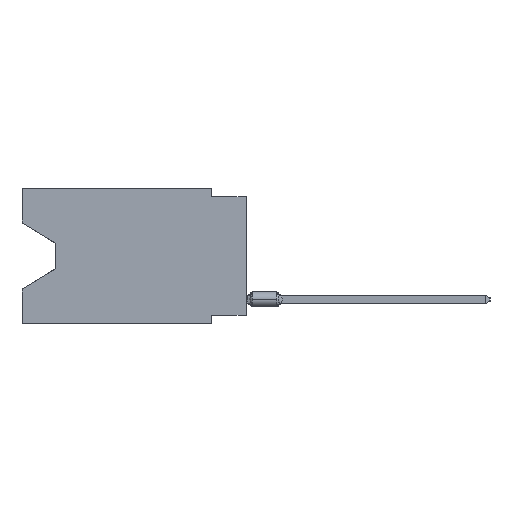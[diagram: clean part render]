
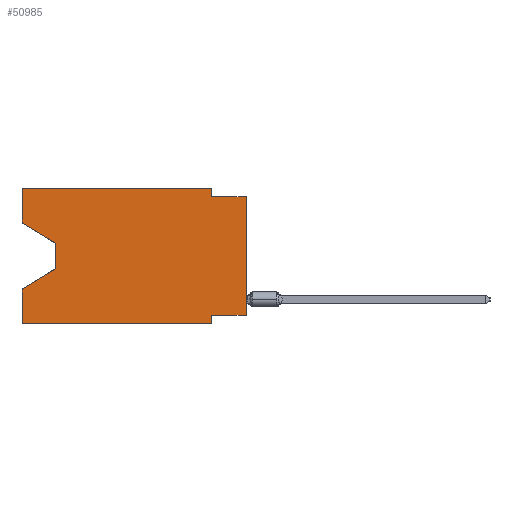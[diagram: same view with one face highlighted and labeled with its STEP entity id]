
A CAD part, left-side view. The second image highlights one B-rep face of the part: STEP entity #50985.
In plain terms, the highlighted planar face has unit normal (-1, 0, 0).
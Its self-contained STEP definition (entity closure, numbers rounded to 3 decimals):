
#1120 = CARTESIAN_POINT ( 'NONE',  ( 0., 0., -9.271 ) ) ;
#1254 = CARTESIAN_POINT ( 'NONE',  ( 0., 13.97, -4.013 ) ) ;
#1329 = EDGE_CURVE ( 'NONE', #47674, #13410, #23877, .T. ) ;
#2119 = EDGE_CURVE ( 'NONE', #50787, #13418, #16677, .T. ) ;
#3861 = EDGE_CURVE ( 'NONE', #7857, #56292, #45244, .T. ) ;
#4808 = VERTEX_POINT ( 'NONE', #8250 ) ;
#4958 = LINE ( 'NONE', #19090, #44811 ) ;
#6176 = ORIENTED_EDGE ( 'NONE', *, *, #52317, .T. ) ;
#6295 = DIRECTION ( 'NONE',  ( 0., 0., -1. ) ) ;
#6825 = VECTOR ( 'NONE', #29955, 1000. ) ;
#6842 = VECTOR ( 'NONE', #49195, 1000. ) ;
#7322 = DIRECTION ( 'NONE',  ( 0., -1., 0. ) ) ;
#7857 = VERTEX_POINT ( 'NONE', #1254 ) ;
#8250 = CARTESIAN_POINT ( 'NONE',  ( 0., 16.383, -7.36 ) ) ;
#8367 = CARTESIAN_POINT ( 'NONE',  ( 0., 16.383, 0. ) ) ;
#8553 = EDGE_CURVE ( 'NONE', #48739, #59104, #13150, .T. ) ;
#12864 = CARTESIAN_POINT ( 'NONE',  ( 0., 2.54, -9.906 ) ) ;
#13150 = LINE ( 'NONE', #26350, #45470 ) ;
#13410 = VERTEX_POINT ( 'NONE', #18545 ) ;
#13416 = EDGE_CURVE ( 'NONE', #17026, #50787, #36682, .T. ) ;
#13418 = VERTEX_POINT ( 'NONE', #55696 ) ;
#13760 = ORIENTED_EDGE ( 'NONE', *, *, #13416, .F. ) ;
#14094 = ORIENTED_EDGE ( 'NONE', *, *, #1329, .F. ) ;
#14321 = ORIENTED_EDGE ( 'NONE', *, *, #29602, .T. ) ;
#15117 = ORIENTED_EDGE ( 'NONE', *, *, #2119, .F. ) ;
#15806 = CARTESIAN_POINT ( 'NONE',  ( 0., 2.54, 0. ) ) ;
#16075 = CARTESIAN_POINT ( 'NONE',  ( 0., 0., -0.635 ) ) ;
#16677 = LINE ( 'NONE', #35412, #44187 ) ;
#16695 = ORIENTED_EDGE ( 'NONE', *, *, #55230, .F. ) ;
#17026 = VERTEX_POINT ( 'NONE', #28528 ) ;
#17269 = FACE_OUTER_BOUND ( 'NONE', #46943, .T. ) ;
#17355 = DIRECTION ( 'NONE',  ( 0., 0., 1. ) ) ;
#18545 = CARTESIAN_POINT ( 'NONE',  ( 0., 2.54, -9.271 ) ) ;
#19090 = CARTESIAN_POINT ( 'NONE',  ( 0., 13.97, -5.893 ) ) ;
#20182 = CARTESIAN_POINT ( 'NONE',  ( 0., 0., -9.271 ) ) ;
#21073 = VERTEX_POINT ( 'NONE', #29047 ) ;
#21563 = CARTESIAN_POINT ( 'NONE',  ( 0., 16.383, -9.906 ) ) ;
#21659 = CARTESIAN_POINT ( 'NONE',  ( 0., 0., 0. ) ) ;
#22740 = LINE ( 'NONE', #31956, #55674 ) ;
#22814 = VECTOR ( 'NONE', #35097, 1000. ) ;
#23416 = ORIENTED_EDGE ( 'NONE', *, *, #8553, .F. ) ;
#23706 = DIRECTION ( 'NONE',  ( 0., 0.855, -0.519 ) ) ;
#23877 = LINE ( 'NONE', #1120, #52016 ) ;
#24664 = EDGE_CURVE ( 'NONE', #13410, #45061, #54695, .T. ) ;
#25677 = ORIENTED_EDGE ( 'NONE', *, *, #56377, .F. ) ;
#26350 = CARTESIAN_POINT ( 'NONE',  ( 0., 0., -0.635 ) ) ;
#26472 = ORIENTED_EDGE ( 'NONE', *, *, #24664, .F. ) ;
#27853 = ORIENTED_EDGE ( 'NONE', *, *, #3861, .T. ) ;
#28528 = CARTESIAN_POINT ( 'NONE',  ( 0., 16.383, -2.546 ) ) ;
#28700 = ORIENTED_EDGE ( 'NONE', *, *, #33602, .T. ) ;
#29047 = CARTESIAN_POINT ( 'NONE',  ( 0., 16.383, -9.906 ) ) ;
#29489 = ORIENTED_EDGE ( 'NONE', *, *, #46172, .T. ) ;
#29602 = EDGE_CURVE ( 'NONE', #47674, #59104, #40690, .T. ) ;
#29955 = DIRECTION ( 'NONE',  ( 0., 0., 1. ) ) ;
#29993 = AXIS2_PLACEMENT_3D ( 'NONE', #8367, #45825, #50723 ) ;
#31372 = CARTESIAN_POINT ( 'NONE',  ( 0., 2.54, -9.906 ) ) ;
#31956 = CARTESIAN_POINT ( 'NONE',  ( 0., 16.383, -2.546 ) ) ;
#33602 = EDGE_CURVE ( 'NONE', #21073, #45061, #58722, .T. ) ;
#34250 = LINE ( 'NONE', #52953, #6825 ) ;
#35078 = CARTESIAN_POINT ( 'NONE',  ( 0., 16.383, 0. ) ) ;
#35097 = DIRECTION ( 'NONE',  ( 0., 0., -1. ) ) ;
#35412 = CARTESIAN_POINT ( 'NONE',  ( 0., 16.383, 0. ) ) ;
#36069 = DIRECTION ( 'NONE',  ( 0., 0., 1. ) ) ;
#36549 = DIRECTION ( 'NONE',  ( 0., -0.855, -0.519 ) ) ;
#36682 = LINE ( 'NONE', #54789, #51841 ) ;
#38484 = VECTOR ( 'NONE', #50092, 1000. ) ;
#38550 = CARTESIAN_POINT ( 'NONE',  ( 0., 13.97, -5.893 ) ) ;
#40690 = LINE ( 'NONE', #21659, #56416 ) ;
#40893 = PLANE ( 'NONE',  #29993 ) ;
#41490 = CARTESIAN_POINT ( 'NONE',  ( 0., 2.54, -0.635 ) ) ;
#42286 = DIRECTION ( 'NONE',  ( 0., 1., 0. ) ) ;
#44187 = VECTOR ( 'NONE', #55952, 1000. ) ;
#44811 = VECTOR ( 'NONE', #23706, 1000. ) ;
#45061 = VERTEX_POINT ( 'NONE', #12864 ) ;
#45070 = VECTOR ( 'NONE', #6295, 1000. ) ;
#45244 = LINE ( 'NONE', #58746, #22814 ) ;
#45470 = VECTOR ( 'NONE', #7322, 1000. ) ;
#45825 = DIRECTION ( 'NONE',  ( 1., 0., 0. ) ) ;
#46172 = EDGE_CURVE ( 'NONE', #17026, #7857, #22740, .T. ) ;
#46943 = EDGE_LOOP ( 'NONE', ( #29489, #27853, #6176, #25677, #28700, #26472, #14094, #14321, #23416, #16695, #15117, #13760 ) ) ;
#47674 = VERTEX_POINT ( 'NONE', #20182 ) ;
#48739 = VERTEX_POINT ( 'NONE', #41490 ) ;
#49195 = DIRECTION ( 'NONE',  ( 0., -1., 0. ) ) ;
#50092 = DIRECTION ( 'NONE',  ( 0., 0., -1. ) ) ;
#50723 = DIRECTION ( 'NONE',  ( 0., 0., -1. ) ) ;
#50787 = VERTEX_POINT ( 'NONE', #35078 ) ;
#50985 = ADVANCED_FACE ( 'NONE', ( #17269 ), #40893, .F. ) ;
#51841 = VECTOR ( 'NONE', #36069, 1000. ) ;
#52016 = VECTOR ( 'NONE', #42286, 1000. ) ;
#52317 = EDGE_CURVE ( 'NONE', #56292, #4808, #4958, .T. ) ;
#52953 = CARTESIAN_POINT ( 'NONE',  ( 0., 16.383, 0. ) ) ;
#54695 = LINE ( 'NONE', #31372, #38484 ) ;
#54789 = CARTESIAN_POINT ( 'NONE',  ( 0., 16.383, 0. ) ) ;
#55230 = EDGE_CURVE ( 'NONE', #13418, #48739, #57877, .T. ) ;
#55674 = VECTOR ( 'NONE', #36549, 1000. ) ;
#55696 = CARTESIAN_POINT ( 'NONE',  ( 0., 2.54, 0. ) ) ;
#55952 = DIRECTION ( 'NONE',  ( 0., -1., 0. ) ) ;
#56292 = VERTEX_POINT ( 'NONE', #38550 ) ;
#56377 = EDGE_CURVE ( 'NONE', #21073, #4808, #34250, .T. ) ;
#56416 = VECTOR ( 'NONE', #17355, 1000. ) ;
#57877 = LINE ( 'NONE', #15806, #45070 ) ;
#58722 = LINE ( 'NONE', #21563, #6842 ) ;
#58746 = CARTESIAN_POINT ( 'NONE',  ( 0., 13.97, -4.013 ) ) ;
#59104 = VERTEX_POINT ( 'NONE', #16075 ) ;
